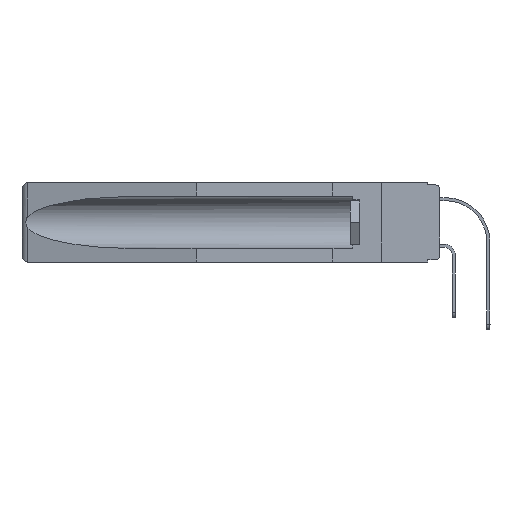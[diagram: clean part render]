
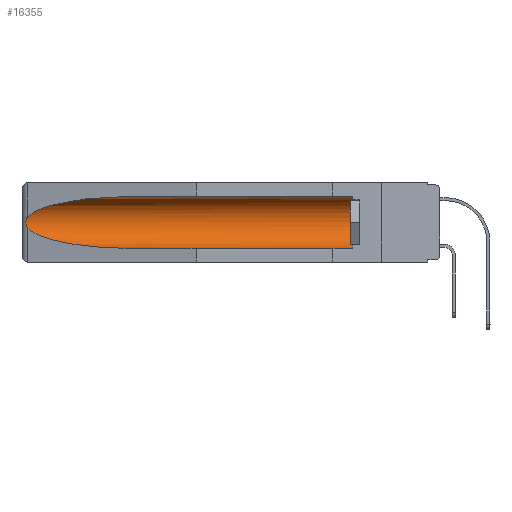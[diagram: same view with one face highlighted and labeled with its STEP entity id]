
A CAD part, left-side view. The second image highlights one B-rep face of the part: STEP entity #16355.
In plain terms, the highlighted cylindrical face has radius 2.857 mm (diameter 5.715 mm), a partial arc.
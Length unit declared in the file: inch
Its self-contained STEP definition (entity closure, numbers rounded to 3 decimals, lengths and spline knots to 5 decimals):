
#54 = EDGE_CURVE ( 'NONE', #476, #9571, #13364, .T. ) ;
#119 = CARTESIAN_POINT ( 'NONE',  ( 0.2673, 1.5327, -0.16383 ) ) ;
#476 = VERTEX_POINT ( 'NONE', #11231 ) ;
#590 = DIRECTION ( 'NONE',  ( 0., 0., 1. ) ) ;
#1187 = CARTESIAN_POINT ( 'NONE',  ( 0.25451, 1.48313, -0.09465 ) ) ;
#1731 = CARTESIAN_POINT ( 'NONE',  ( 0.26537, 1.52718, -0.19328 ) ) ;
#2128 = VECTOR ( 'NONE', #20402, 39.37008 ) ;
#2473 = ORIENTED_EDGE ( 'NONE', *, *, #6268, .T. ) ;
#2604 = CARTESIAN_POINT ( 'NONE',  ( 0.26537, 1.52718, -0.14972 ) ) ;
#2926 = VERTEX_POINT ( 'NONE', #9186 ) ;
#4258 = CARTESIAN_POINT ( 'NONE',  ( 0.155, 0.126, -0.1715 ) ) ;
#4766 = CARTESIAN_POINT ( 'NONE',  ( 0.26655, 1.53094, -0.18657 ) ) ;
#4822 = CARTESIAN_POINT ( 'NONE',  ( 0.155, 0.126, -0.284 ) ) ;
#4983 = CARTESIAN_POINT ( 'NONE',  ( 0.2675, 1.53308, -0.17534 ) ) ;
#5585 = VERTEX_POINT ( 'NONE', #20241 ) ;
#5787 = LINE ( 'NONE', #20681, #10743 ) ;
#5978 = VERTEX_POINT ( 'NONE', #4822 ) ;
#6139 = CARTESIAN_POINT ( 'NONE',  ( 0.155, -0.30754, -0.1715 ) ) ;
#6219 = EDGE_CURVE ( 'NONE', #5978, #5585, #5787, .T. ) ;
#6268 = EDGE_CURVE ( 'NONE', #5978, #2926, #9029, .T. ) ;
#6351 = DIRECTION ( 'NONE',  ( 0., 0., 1. ) ) ;
#6356 = CARTESIAN_POINT ( 'NONE',  ( 0.26537, 1.52718, -0.19328 ) ) ;
#6618 = CARTESIAN_POINT ( 'NONE',  ( 0.26537, 1.52718, -0.19328 ) ) ;
#6791 = EDGE_CURVE ( 'NONE', #11099, #476, #16844, .T. ) ;
#6953 = AXIS2_PLACEMENT_3D ( 'NONE', #4258, #10852, #590 ) ;
#7145 = ORIENTED_EDGE ( 'NONE', *, *, #7193, .T. ) ;
#7193 = EDGE_CURVE ( 'NONE', #2926, #11099, #15961, .T. ) ;
#8835 = CARTESIAN_POINT ( 'NONE',  ( 0.155, 1.07973, -0.059 ) ) ;
#9029 = CIRCLE ( 'NONE', #6953, 0.1125 ) ;
#9186 = CARTESIAN_POINT ( 'NONE',  ( 0.155, 0.126, -0.059 ) ) ;
#9571 = VERTEX_POINT ( 'NONE', #6618 ) ;
#9713 = CARTESIAN_POINT ( 'NONE',  ( 0.21114, 1.30732, -0.284 ) ) ;
#9846 = CARTESIAN_POINT ( 'NONE',  ( 0.2675, 1.53308, -0.16763 ) ) ;
#10743 = VECTOR ( 'NONE', #19072, 39.37008 ) ;
#10831 = CARTESIAN_POINT ( 'NONE',  ( 0.155, 1.07973, -0.059 ) ) ;
#10852 = DIRECTION ( 'NONE',  ( 0., -1., 0. ) ) ;
#11099 = VERTEX_POINT ( 'NONE', #8835 ) ;
#11231 = CARTESIAN_POINT ( 'NONE',  ( 0.26537, 1.52718, -0.14972 ) ) ;
#11327 = CYLINDRICAL_SURFACE ( 'NONE', #17870, 0.1125 ) ;
#11361 = CARTESIAN_POINT ( 'NONE',  ( 0.26597, 1.5296, -0.19026 ) ) ;
#11701 = CARTESIAN_POINT ( 'NONE',  ( 0.2673, 1.53269, -0.17917 ) ) ;
#12753 = ORIENTED_EDGE ( 'NONE', *, *, #6791, .T. ) ;
#13364 = B_SPLINE_CURVE_WITH_KNOTS ( 'NONE', 3,
 ( #18762, #17515, #17830, #119, #9846, #4983, #11701, #4766, #11361, #1731 ),
 .UNSPECIFIED., .F., .F.,
 ( 4, 2, 2, 2, 4 ),
 ( 0., 0.00029, 0.00058, 0.00087, 0.00117 ),
 .UNSPECIFIED. ) ;
#13832 = CARTESIAN_POINT ( 'NONE',  ( 0.155, -0.30754, -0.059 ) ) ;
#13981 = EDGE_CURVE ( 'NONE', #9571, #5585, #21246, .T. ) ;
#14418 = ORIENTED_EDGE ( 'NONE', *, *, #54, .T. ) ;
#14673 = FACE_OUTER_BOUND ( 'NONE', #21212, .T. ) ;
#15799 = CARTESIAN_POINT ( 'NONE',  ( 0.21114, 1.30732, -0.059 ) ) ;
#15961 = LINE ( 'NONE', #13832, #2128 ) ;
#16294 = CARTESIAN_POINT ( 'NONE',  ( 0.155, 1.07973, -0.284 ) ) ;
#16355 = ADVANCED_FACE ( 'NONE', ( #14673 ), #11327, .F. ) ;
#16844 =( BOUNDED_CURVE ( )  B_SPLINE_CURVE ( 3, ( #10831, #15799, #1187, #2604 ),
 .UNSPECIFIED., .F., .T. ) 
 B_SPLINE_CURVE_WITH_KNOTS ( ( 4, 4 ),
 ( 4.71239, 6.08839 ),
 .UNSPECIFIED. ) 
 CURVE ( )  GEOMETRIC_REPRESENTATION_ITEM ( )  RATIONAL_B_SPLINE_CURVE ( ( 1., 0.848, 0.848, 1. ) ) 
 REPRESENTATION_ITEM ( '' )  );
#17515 = CARTESIAN_POINT ( 'NONE',  ( 0.26597, 1.52961, -0.15275 ) ) ;
#17830 = CARTESIAN_POINT ( 'NONE',  ( 0.26654, 1.53092, -0.15636 ) ) ;
#17870 = AXIS2_PLACEMENT_3D ( 'NONE', #6139, #21152, #6351 ) ;
#17918 = CARTESIAN_POINT ( 'NONE',  ( 0.25451, 1.48313, -0.24835 ) ) ;
#18762 = CARTESIAN_POINT ( 'NONE',  ( 0.26537, 1.52718, -0.14972 ) ) ;
#19072 = DIRECTION ( 'NONE',  ( 0., 1., 0. ) ) ;
#19936 = ORIENTED_EDGE ( 'NONE', *, *, #6219, .F. ) ;
#20241 = CARTESIAN_POINT ( 'NONE',  ( 0.155, 1.07973, -0.284 ) ) ;
#20402 = DIRECTION ( 'NONE',  ( 0., 1., 0. ) ) ;
#20681 = CARTESIAN_POINT ( 'NONE',  ( 0.155, -0.30754, -0.284 ) ) ;
#21091 = ORIENTED_EDGE ( 'NONE', *, *, #13981, .T. ) ;
#21152 = DIRECTION ( 'NONE',  ( 0., 1., 0. ) ) ;
#21212 = EDGE_LOOP ( 'NONE', ( #12753, #14418, #21091, #19936, #2473, #7145 ) ) ;
#21246 =( BOUNDED_CURVE ( )  B_SPLINE_CURVE ( 3, ( #6356, #17918, #9713, #16294 ),
 .UNSPECIFIED., .F., .T. ) 
 B_SPLINE_CURVE_WITH_KNOTS ( ( 4, 4 ),
 ( 0.1948, 1.5708 ),
 .UNSPECIFIED. ) 
 CURVE ( )  GEOMETRIC_REPRESENTATION_ITEM ( )  RATIONAL_B_SPLINE_CURVE ( ( 1., 0.848, 0.848, 1. ) ) 
 REPRESENTATION_ITEM ( '' )  );
